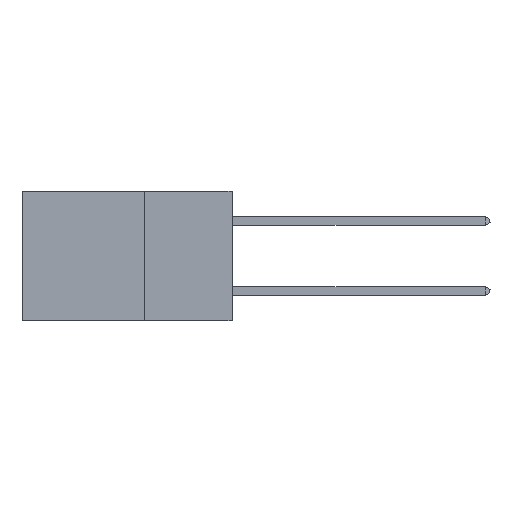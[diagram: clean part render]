
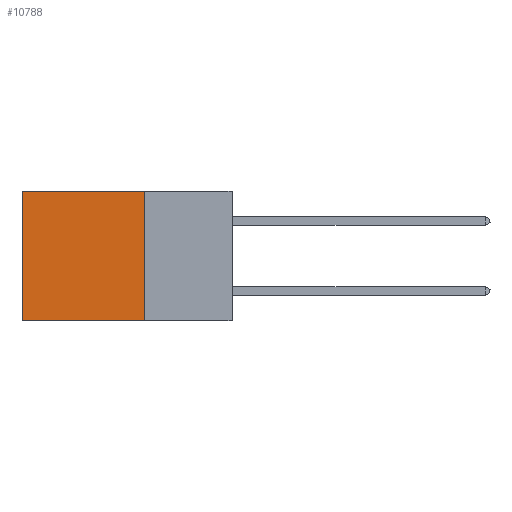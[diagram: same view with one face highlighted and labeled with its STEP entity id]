
A CAD part, left-side view. The second image highlights one B-rep face of the part: STEP entity #10788.
In plain terms, the highlighted planar face has unit normal (-1, 0, 0).
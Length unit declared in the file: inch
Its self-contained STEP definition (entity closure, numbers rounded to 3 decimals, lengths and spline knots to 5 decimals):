
#213 = VERTEX_POINT ( 'NONE', #19956 ) ;
#1889 = LINE ( 'NONE', #21194, #8940 ) ;
#2078 = DIRECTION ( 'NONE',  ( 0., 0., -1. ) ) ;
#2697 = ORIENTED_EDGE ( 'NONE', *, *, #17728, .T. ) ;
#3059 = CARTESIAN_POINT ( 'NONE',  ( 0.2875, 0.6, 0. ) ) ;
#3321 = DIRECTION ( 'NONE',  ( 1., 0., 0. ) ) ;
#3414 = ORIENTED_EDGE ( 'NONE', *, *, #24158, .F. ) ;
#4667 = DIRECTION ( 'NONE',  ( 0., 1., 0. ) ) ;
#4921 = LINE ( 'NONE', #3059, #29548 ) ;
#5026 = EDGE_LOOP ( 'NONE', ( #2697, #3414, #7690, #27908 ) ) ;
#5390 = VERTEX_POINT ( 'NONE', #24661 ) ;
#5555 = VECTOR ( 'NONE', #8210, 39.37008 ) ;
#5719 = AXIS2_PLACEMENT_3D ( 'NONE', #13300, #3321, #2078 ) ;
#7690 = ORIENTED_EDGE ( 'NONE', *, *, #29970, .F. ) ;
#7827 = DIRECTION ( 'NONE',  ( 0., 0., -1. ) ) ;
#8136 = CARTESIAN_POINT ( 'NONE',  ( 0.2875, 0.6, 0. ) ) ;
#8210 = DIRECTION ( 'NONE',  ( 0., 1., 0. ) ) ;
#8913 = LINE ( 'NONE', #18976, #23473 ) ;
#8940 = VECTOR ( 'NONE', #16664, 39.37008 ) ;
#10628 = CARTESIAN_POINT ( 'NONE',  ( 0.2875, 0.25, 0. ) ) ;
#10788 = ADVANCED_FACE ( 'NONE', ( #21065 ), #13514, .F. ) ;
#11933 = LINE ( 'NONE', #10628, #5555 ) ;
#13300 = CARTESIAN_POINT ( 'NONE',  ( 0.2875, 0.25, 0. ) ) ;
#13514 = PLANE ( 'NONE',  #5719 ) ;
#16664 = DIRECTION ( 'NONE',  ( 0., 0., -1. ) ) ;
#17728 = EDGE_CURVE ( 'NONE', #25187, #25074, #4921, .T. ) ;
#18976 = CARTESIAN_POINT ( 'NONE',  ( 0.2875, 0.25, -0.37 ) ) ;
#19956 = CARTESIAN_POINT ( 'NONE',  ( 0.2875, 0.25, -0.37 ) ) ;
#21065 = FACE_OUTER_BOUND ( 'NONE', #5026, .T. ) ;
#21194 = CARTESIAN_POINT ( 'NONE',  ( 0.2875, 0.25, 0. ) ) ;
#23473 = VECTOR ( 'NONE', #4667, 39.37008 ) ;
#24158 = EDGE_CURVE ( 'NONE', #213, #25074, #8913, .T. ) ;
#24661 = CARTESIAN_POINT ( 'NONE',  ( 0.2875, 0.25, 0. ) ) ;
#25074 = VERTEX_POINT ( 'NONE', #26654 ) ;
#25187 = VERTEX_POINT ( 'NONE', #8136 ) ;
#26654 = CARTESIAN_POINT ( 'NONE',  ( 0.2875, 0.6, -0.37 ) ) ;
#27908 = ORIENTED_EDGE ( 'NONE', *, *, #30349, .T. ) ;
#29548 = VECTOR ( 'NONE', #7827, 39.37008 ) ;
#29970 = EDGE_CURVE ( 'NONE', #5390, #213, #1889, .T. ) ;
#30349 = EDGE_CURVE ( 'NONE', #5390, #25187, #11933, .T. ) ;
